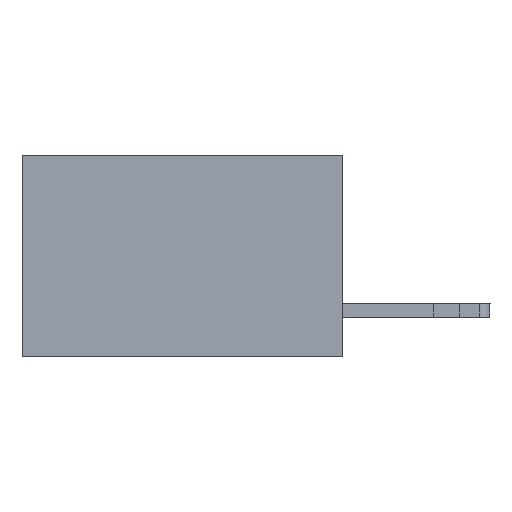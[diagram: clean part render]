
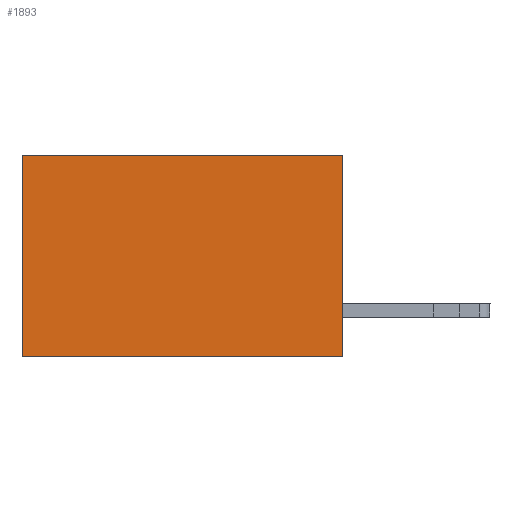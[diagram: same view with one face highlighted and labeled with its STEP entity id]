
A CAD part, left-side view. The second image highlights one B-rep face of the part: STEP entity #1893.
In plain terms, the highlighted planar face has unit normal (-1, 0, 0).
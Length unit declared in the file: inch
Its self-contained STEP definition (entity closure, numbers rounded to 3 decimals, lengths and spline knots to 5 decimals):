
#6 = EDGE_CURVE ( 'NONE', #1785, #14045, #9002, .T. ) ;
#916 = EDGE_LOOP ( 'NONE', ( #10501, #8393, #5895, #9911 ) ) ;
#1785 = VERTEX_POINT ( 'NONE', #2803 ) ;
#1893 = ADVANCED_FACE ( 'NONE', ( #4494 ), #6613, .F. ) ;
#1912 = DIRECTION ( 'NONE',  ( 0., 0., -1. ) ) ;
#2100 = EDGE_CURVE ( 'NONE', #6196, #14045, #3865, .T. ) ;
#2803 = CARTESIAN_POINT ( 'NONE',  ( 0.277, 0.59, 0. ) ) ;
#3584 = VERTEX_POINT ( 'NONE', #4792 ) ;
#3865 = LINE ( 'NONE', #10822, #10076 ) ;
#4475 = DIRECTION ( 'NONE',  ( 0., 0., -1. ) ) ;
#4494 = FACE_OUTER_BOUND ( 'NONE', #916, .T. ) ;
#4792 = CARTESIAN_POINT ( 'NONE',  ( 0.277, 0., 0. ) ) ;
#5278 = EDGE_CURVE ( 'NONE', #3584, #1785, #8812, .T. ) ;
#5400 = CARTESIAN_POINT ( 'NONE',  ( 0.277, 0.59, -0.37 ) ) ;
#5736 = VECTOR ( 'NONE', #1912, 39.37008 ) ;
#5895 = ORIENTED_EDGE ( 'NONE', *, *, #6092, .F. ) ;
#5905 = CARTESIAN_POINT ( 'NONE',  ( 0.277, 0.59, -0.37 ) ) ;
#6092 = EDGE_CURVE ( 'NONE', #3584, #6196, #9555, .T. ) ;
#6196 = VERTEX_POINT ( 'NONE', #9474 ) ;
#6613 = PLANE ( 'NONE',  #7679 ) ;
#6630 = DIRECTION ( 'NONE',  ( 1., 0., 0. ) ) ;
#7679 = AXIS2_PLACEMENT_3D ( 'NONE', #15642, #6630, #4475 ) ;
#8393 = ORIENTED_EDGE ( 'NONE', *, *, #2100, .F. ) ;
#8812 = LINE ( 'NONE', #9415, #15304 ) ;
#9002 = LINE ( 'NONE', #5400, #5736 ) ;
#9384 = DIRECTION ( 'NONE',  ( 0., 1., 0. ) ) ;
#9415 = CARTESIAN_POINT ( 'NONE',  ( 0.277, 0., 0. ) ) ;
#9474 = CARTESIAN_POINT ( 'NONE',  ( 0.277, 0., -0.37 ) ) ;
#9555 = LINE ( 'NONE', #11192, #15647 ) ;
#9911 = ORIENTED_EDGE ( 'NONE', *, *, #5278, .T. ) ;
#10076 = VECTOR ( 'NONE', #13888, 39.37008 ) ;
#10501 = ORIENTED_EDGE ( 'NONE', *, *, #6, .T. ) ;
#10822 = CARTESIAN_POINT ( 'NONE',  ( 0.277, 0., -0.37 ) ) ;
#10849 = DIRECTION ( 'NONE',  ( 0., 0., -1. ) ) ;
#11192 = CARTESIAN_POINT ( 'NONE',  ( 0.277, 0., -0.37 ) ) ;
#13888 = DIRECTION ( 'NONE',  ( 0., 1., 0. ) ) ;
#14045 = VERTEX_POINT ( 'NONE', #5905 ) ;
#15304 = VECTOR ( 'NONE', #9384, 39.37008 ) ;
#15642 = CARTESIAN_POINT ( 'NONE',  ( 0.277, 0., -0.37 ) ) ;
#15647 = VECTOR ( 'NONE', #10849, 39.37008 ) ;
